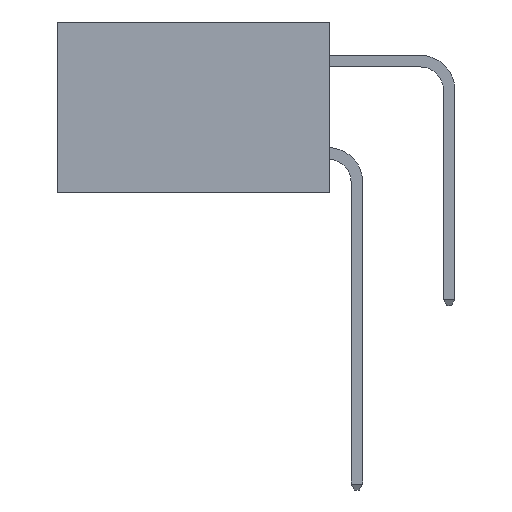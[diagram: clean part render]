
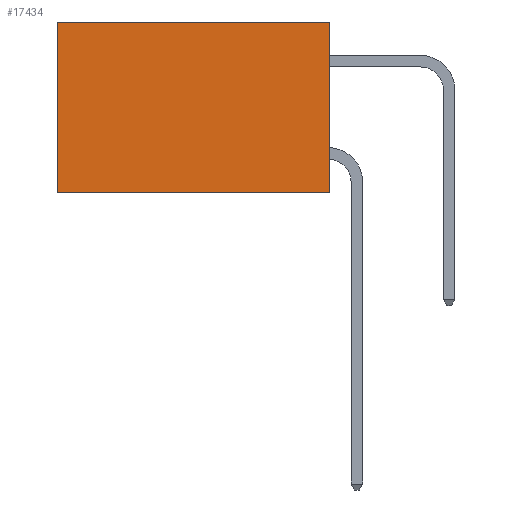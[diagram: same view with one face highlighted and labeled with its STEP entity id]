
A CAD part, left-side view. The second image highlights one B-rep face of the part: STEP entity #17434.
In plain terms, the highlighted planar face has unit normal (-1, 0, 0).
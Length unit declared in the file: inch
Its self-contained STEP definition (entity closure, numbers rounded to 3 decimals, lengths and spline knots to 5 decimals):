
#1235 = CARTESIAN_POINT ( 'NONE',  ( 0.277, 0.59, -0.37 ) ) ;
#2340 = ORIENTED_EDGE ( 'NONE', *, *, #22891, .F. ) ;
#2374 = CARTESIAN_POINT ( 'NONE',  ( 0.277, 0., 0. ) ) ;
#2756 = VECTOR ( 'NONE', #3279, 39.37008 ) ;
#3279 = DIRECTION ( 'NONE',  ( 0., 0., -1. ) ) ;
#3972 = CARTESIAN_POINT ( 'NONE',  ( 0.277, 0., -0.37 ) ) ;
#4585 = CARTESIAN_POINT ( 'NONE',  ( 0.277, 0., 0. ) ) ;
#5652 = VERTEX_POINT ( 'NONE', #11476 ) ;
#5748 = ORIENTED_EDGE ( 'NONE', *, *, #18822, .T. ) ;
#6273 = CARTESIAN_POINT ( 'NONE',  ( 0.277, 0., -0.37 ) ) ;
#7611 = EDGE_LOOP ( 'NONE', ( #12634, #2340, #15795, #5748 ) ) ;
#7672 = EDGE_CURVE ( 'NONE', #5652, #22434, #22893, .T. ) ;
#8287 = DIRECTION ( 'NONE',  ( 1., 0., 0. ) ) ;
#9810 = FACE_OUTER_BOUND ( 'NONE', #7611, .T. ) ;
#9922 = CARTESIAN_POINT ( 'NONE',  ( 0.277, 0., -0.37 ) ) ;
#11476 = CARTESIAN_POINT ( 'NONE',  ( 0.277, 0.59, 0. ) ) ;
#12634 = ORIENTED_EDGE ( 'NONE', *, *, #7672, .T. ) ;
#13530 = CARTESIAN_POINT ( 'NONE',  ( 0.277, 0., -0.37 ) ) ;
#13692 = DIRECTION ( 'NONE',  ( 0., 1., 0. ) ) ;
#14534 = VECTOR ( 'NONE', #19441, 39.37008 ) ;
#15403 = VECTOR ( 'NONE', #16262, 39.37008 ) ;
#15795 = ORIENTED_EDGE ( 'NONE', *, *, #18555, .F. ) ;
#16262 = DIRECTION ( 'NONE',  ( 0., 1., 0. ) ) ;
#17434 = ADVANCED_FACE ( 'NONE', ( #9810 ), #17806, .F. ) ;
#17661 = AXIS2_PLACEMENT_3D ( 'NONE', #6273, #8287, #21688 ) ;
#17806 = PLANE ( 'NONE',  #17661 ) ;
#18555 = EDGE_CURVE ( 'NONE', #24942, #20450, #20238, .T. ) ;
#18822 = EDGE_CURVE ( 'NONE', #24942, #5652, #21102, .T. ) ;
#19441 = DIRECTION ( 'NONE',  ( 0., 0., -1. ) ) ;
#20030 = VECTOR ( 'NONE', #13692, 39.37008 ) ;
#20238 = LINE ( 'NONE', #9922, #14534 ) ;
#20450 = VERTEX_POINT ( 'NONE', #13530 ) ;
#21102 = LINE ( 'NONE', #4585, #15403 ) ;
#21688 = DIRECTION ( 'NONE',  ( 0., 0., -1. ) ) ;
#22434 = VERTEX_POINT ( 'NONE', #25117 ) ;
#22891 = EDGE_CURVE ( 'NONE', #20450, #22434, #24562, .T. ) ;
#22893 = LINE ( 'NONE', #1235, #2756 ) ;
#24562 = LINE ( 'NONE', #3972, #20030 ) ;
#24942 = VERTEX_POINT ( 'NONE', #2374 ) ;
#25117 = CARTESIAN_POINT ( 'NONE',  ( 0.277, 0.59, -0.37 ) ) ;
